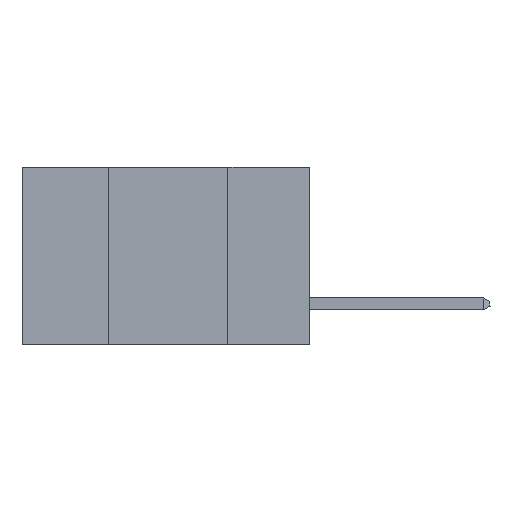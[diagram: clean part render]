
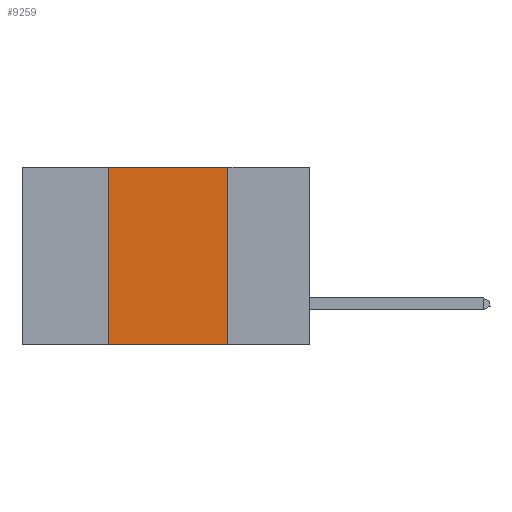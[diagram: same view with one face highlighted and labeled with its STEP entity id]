
A CAD part, left-side view. The second image highlights one B-rep face of the part: STEP entity #9259.
In plain terms, the highlighted planar face has unit normal (-1, 0, 0).
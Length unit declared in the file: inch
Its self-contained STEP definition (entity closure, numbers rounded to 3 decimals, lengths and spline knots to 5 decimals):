
#799 = DIRECTION ( 'NONE',  ( 0., -1., 0. ) ) ;
#1423 = CARTESIAN_POINT ( 'NONE',  ( 0., 0.42, 0. ) ) ;
#2509 = ORIENTED_EDGE ( 'NONE', *, *, #14305, .F. ) ;
#3224 = VECTOR ( 'NONE', #8362, 39.37008 ) ;
#4744 = VECTOR ( 'NONE', #799, 39.37008 ) ;
#5135 = LINE ( 'NONE', #1423, #22042 ) ;
#5979 = CARTESIAN_POINT ( 'NONE',  ( 0., 0.6, 0. ) ) ;
#6751 = FACE_OUTER_BOUND ( 'NONE', #34407, .T. ) ;
#8362 = DIRECTION ( 'NONE',  ( 0., -1., 0. ) ) ;
#9259 = ADVANCED_FACE ( 'NONE', ( #6751 ), #31349, .F. ) ;
#11523 = LINE ( 'NONE', #40066, #4744 ) ;
#13008 = EDGE_CURVE ( 'NONE', #16164, #29852, #11523, .T. ) ;
#14305 = EDGE_CURVE ( 'NONE', #27215, #16164, #5135, .T. ) ;
#14482 = CARTESIAN_POINT ( 'NONE',  ( 0., 0.42, -0.37 ) ) ;
#15644 = CARTESIAN_POINT ( 'NONE',  ( 0., 0.6, -0.37 ) ) ;
#16024 = CARTESIAN_POINT ( 'NONE',  ( 0., 0.17, 0. ) ) ;
#16029 = ORIENTED_EDGE ( 'NONE', *, *, #13008, .F. ) ;
#16164 = VERTEX_POINT ( 'NONE', #31703 ) ;
#17332 = LINE ( 'NONE', #15644, #3224 ) ;
#20310 = ORIENTED_EDGE ( 'NONE', *, *, #35054, .T. ) ;
#22042 = VECTOR ( 'NONE', #44608, 39.37008 ) ;
#22502 = CARTESIAN_POINT ( 'NONE',  ( 0., 0.17, -0.37 ) ) ;
#23111 = DIRECTION ( 'NONE',  ( 0., 0., -1. ) ) ;
#27215 = VERTEX_POINT ( 'NONE', #14482 ) ;
#29852 = VERTEX_POINT ( 'NONE', #44959 ) ;
#30995 = EDGE_CURVE ( 'NONE', #29852, #32101, #33122, .T. ) ;
#31349 = PLANE ( 'NONE',  #35922 ) ;
#31500 = DIRECTION ( 'NONE',  ( 0., 0., -1. ) ) ;
#31703 = CARTESIAN_POINT ( 'NONE',  ( 0., 0.42, 0. ) ) ;
#32101 = VERTEX_POINT ( 'NONE', #22502 ) ;
#33122 = LINE ( 'NONE', #16024, #46542 ) ;
#34407 = EDGE_LOOP ( 'NONE', ( #35663, #16029, #2509, #20310 ) ) ;
#35054 = EDGE_CURVE ( 'NONE', #27215, #32101, #17332, .T. ) ;
#35663 = ORIENTED_EDGE ( 'NONE', *, *, #30995, .F. ) ;
#35922 = AXIS2_PLACEMENT_3D ( 'NONE', #5979, #41934, #31500 ) ;
#40066 = CARTESIAN_POINT ( 'NONE',  ( 0., 0.6, 0. ) ) ;
#41934 = DIRECTION ( 'NONE',  ( 1., 0., 0. ) ) ;
#44608 = DIRECTION ( 'NONE',  ( 0., 0., 1. ) ) ;
#44959 = CARTESIAN_POINT ( 'NONE',  ( 0., 0.17, 0. ) ) ;
#46542 = VECTOR ( 'NONE', #23111, 39.37008 ) ;
